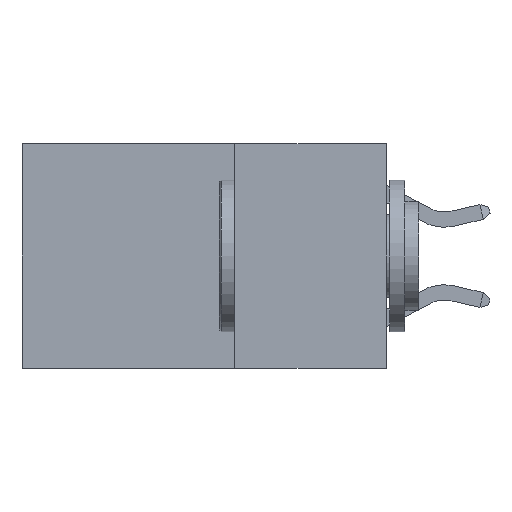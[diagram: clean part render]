
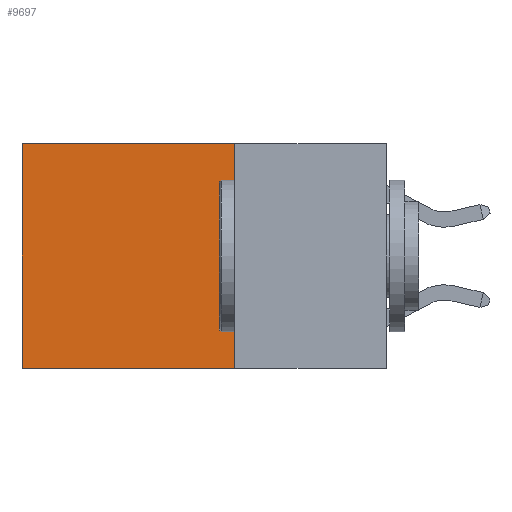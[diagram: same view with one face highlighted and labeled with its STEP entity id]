
A CAD part, left-side view. The second image highlights one B-rep face of the part: STEP entity #9697.
In plain terms, the highlighted planar face has unit normal (-1, 0, 0).
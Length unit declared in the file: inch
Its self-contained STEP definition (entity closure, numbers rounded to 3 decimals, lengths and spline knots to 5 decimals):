
#400 = FACE_OUTER_BOUND ( 'NONE', #7115, .T. ) ;
#773 = ORIENTED_EDGE ( 'NONE', *, *, #9715, .T. ) ;
#986 = ORIENTED_EDGE ( 'NONE', *, *, #5492, .F. ) ;
#1388 = CARTESIAN_POINT ( 'NONE',  ( 0.2625, 0.25, 0. ) ) ;
#1394 = VECTOR ( 'NONE', #2319, 39.37008 ) ;
#1451 = ORIENTED_EDGE ( 'NONE', *, *, #2240, .T. ) ;
#1620 = VERTEX_POINT ( 'NONE', #7232 ) ;
#1807 = ORIENTED_EDGE ( 'NONE', *, *, #3189, .F. ) ;
#2199 = CARTESIAN_POINT ( 'NONE',  ( 0.2625, 0.25, -0.37 ) ) ;
#2240 = EDGE_CURVE ( 'NONE', #5331, #1620, #7384, .T. ) ;
#2319 = DIRECTION ( 'NONE',  ( 0., 0., -1. ) ) ;
#2548 = CARTESIAN_POINT ( 'NONE',  ( 0.2625, 0.25, 0. ) ) ;
#2972 = AXIS2_PLACEMENT_3D ( 'NONE', #2548, #3462, #9300 ) ;
#3142 = VECTOR ( 'NONE', #5773, 39.37008 ) ;
#3150 = VECTOR ( 'NONE', #4362, 39.37008 ) ;
#3189 = EDGE_CURVE ( 'NONE', #5394, #1620, #5413, .T. ) ;
#3462 = DIRECTION ( 'NONE',  ( 1., 0., 0. ) ) ;
#4362 = DIRECTION ( 'NONE',  ( 0., 0., -1. ) ) ;
#4920 = VECTOR ( 'NONE', #6030, 39.37008 ) ;
#5211 = LINE ( 'NONE', #10074, #4920 ) ;
#5331 = VERTEX_POINT ( 'NONE', #6436 ) ;
#5394 = VERTEX_POINT ( 'NONE', #2199 ) ;
#5413 = LINE ( 'NONE', #9852, #3142 ) ;
#5492 = EDGE_CURVE ( 'NONE', #9788, #5394, #8242, .T. ) ;
#5773 = DIRECTION ( 'NONE',  ( 0., 1., 0. ) ) ;
#6030 = DIRECTION ( 'NONE',  ( 0., 1., 0. ) ) ;
#6436 = CARTESIAN_POINT ( 'NONE',  ( 0.2625, 0.6, 0. ) ) ;
#7115 = EDGE_LOOP ( 'NONE', ( #1451, #1807, #986, #773 ) ) ;
#7232 = CARTESIAN_POINT ( 'NONE',  ( 0.2625, 0.6, -0.37 ) ) ;
#7384 = LINE ( 'NONE', #9352, #3150 ) ;
#7673 = PLANE ( 'NONE',  #2972 ) ;
#7779 = CARTESIAN_POINT ( 'NONE',  ( 0.2625, 0.25, 0. ) ) ;
#8242 = LINE ( 'NONE', #1388, #1394 ) ;
#9300 = DIRECTION ( 'NONE',  ( 0., 0., -1. ) ) ;
#9352 = CARTESIAN_POINT ( 'NONE',  ( 0.2625, 0.6, 0. ) ) ;
#9697 = ADVANCED_FACE ( 'NONE', ( #400 ), #7673, .F. ) ;
#9715 = EDGE_CURVE ( 'NONE', #9788, #5331, #5211, .T. ) ;
#9788 = VERTEX_POINT ( 'NONE', #7779 ) ;
#9852 = CARTESIAN_POINT ( 'NONE',  ( 0.2625, 0.25, -0.37 ) ) ;
#10074 = CARTESIAN_POINT ( 'NONE',  ( 0.2625, 0.25, 0. ) ) ;
